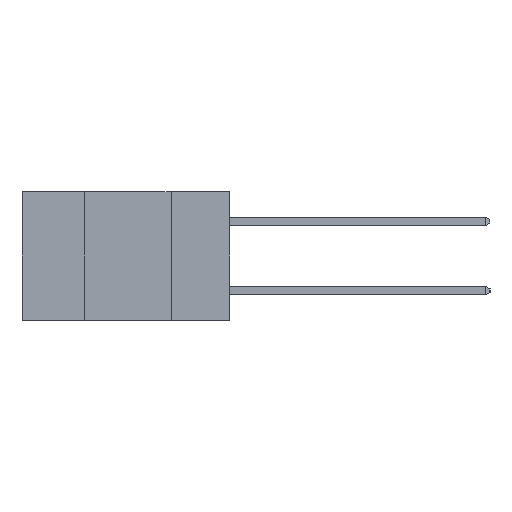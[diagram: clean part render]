
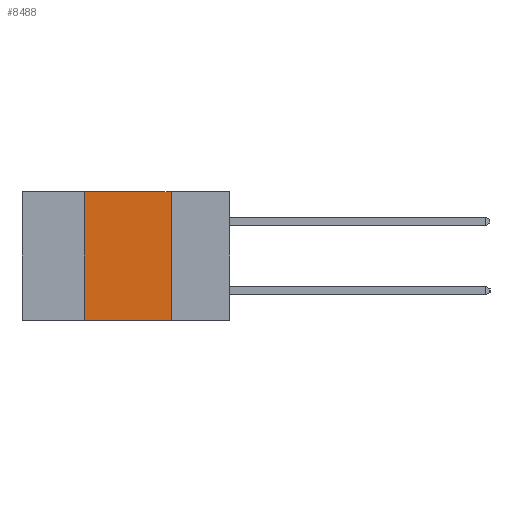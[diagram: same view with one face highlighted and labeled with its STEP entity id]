
A CAD part, left-side view. The second image highlights one B-rep face of the part: STEP entity #8488.
In plain terms, the highlighted planar face has unit normal (-1, 0, 0).
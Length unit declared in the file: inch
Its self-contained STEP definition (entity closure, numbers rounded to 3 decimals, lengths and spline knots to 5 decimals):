
#147 = ORIENTED_EDGE ( 'NONE', *, *, #9615, .T. ) ;
#775 = DIRECTION ( 'NONE',  ( 0., -1., 0. ) ) ;
#929 = VERTEX_POINT ( 'NONE', #9120 ) ;
#1461 = EDGE_CURVE ( 'NONE', #4033, #5467, #4348, .T. ) ;
#1563 = ORIENTED_EDGE ( 'NONE', *, *, #1461, .F. ) ;
#1913 = LINE ( 'NONE', #5904, #11920 ) ;
#2477 = EDGE_LOOP ( 'NONE', ( #10638, #1563, #12831, #147 ) ) ;
#2782 = VERTEX_POINT ( 'NONE', #9282 ) ;
#2841 = DIRECTION ( 'NONE',  ( 0., 0., 1. ) ) ;
#2892 = DIRECTION ( 'NONE',  ( 0., -1., 0. ) ) ;
#3339 = CARTESIAN_POINT ( 'NONE',  ( 0., 0.17, -0.37 ) ) ;
#3922 = DIRECTION ( 'NONE',  ( 0., 0., -1. ) ) ;
#4033 = VERTEX_POINT ( 'NONE', #9931 ) ;
#4219 = EDGE_CURVE ( 'NONE', #5467, #929, #9797, .T. ) ;
#4348 = LINE ( 'NONE', #8892, #7657 ) ;
#4715 = CARTESIAN_POINT ( 'NONE',  ( 0., 0.17, 0. ) ) ;
#5467 = VERTEX_POINT ( 'NONE', #4715 ) ;
#5557 = FACE_OUTER_BOUND ( 'NONE', #2477, .T. ) ;
#5840 = LINE ( 'NONE', #12706, #10837 ) ;
#5904 = CARTESIAN_POINT ( 'NONE',  ( 0., 0.42, -0.37 ) ) ;
#7133 = VECTOR ( 'NONE', #11341, 39.37008 ) ;
#7657 = VECTOR ( 'NONE', #2892, 39.37008 ) ;
#8488 = ADVANCED_FACE ( 'NONE', ( #5557 ), #8896, .F. ) ;
#8892 = CARTESIAN_POINT ( 'NONE',  ( 0., 0.6, 0. ) ) ;
#8896 = PLANE ( 'NONE',  #12657 ) ;
#9120 = CARTESIAN_POINT ( 'NONE',  ( 0., 0.17, -0.37 ) ) ;
#9282 = CARTESIAN_POINT ( 'NONE',  ( 0., 0.42, -0.37 ) ) ;
#9615 = EDGE_CURVE ( 'NONE', #2782, #929, #5840, .T. ) ;
#9797 = LINE ( 'NONE', #3339, #7133 ) ;
#9905 = DIRECTION ( 'NONE',  ( 1., 0., 0. ) ) ;
#9931 = CARTESIAN_POINT ( 'NONE',  ( 0., 0.42, 0. ) ) ;
#10638 = ORIENTED_EDGE ( 'NONE', *, *, #4219, .F. ) ;
#10837 = VECTOR ( 'NONE', #775, 39.37008 ) ;
#11341 = DIRECTION ( 'NONE',  ( 0., 0., -1. ) ) ;
#11817 = CARTESIAN_POINT ( 'NONE',  ( 0., 0.6, 0. ) ) ;
#11920 = VECTOR ( 'NONE', #2841, 39.37008 ) ;
#12347 = EDGE_CURVE ( 'NONE', #2782, #4033, #1913, .T. ) ;
#12657 = AXIS2_PLACEMENT_3D ( 'NONE', #11817, #9905, #3922 ) ;
#12706 = CARTESIAN_POINT ( 'NONE',  ( 0., 0.6, -0.37 ) ) ;
#12831 = ORIENTED_EDGE ( 'NONE', *, *, #12347, .F. ) ;
